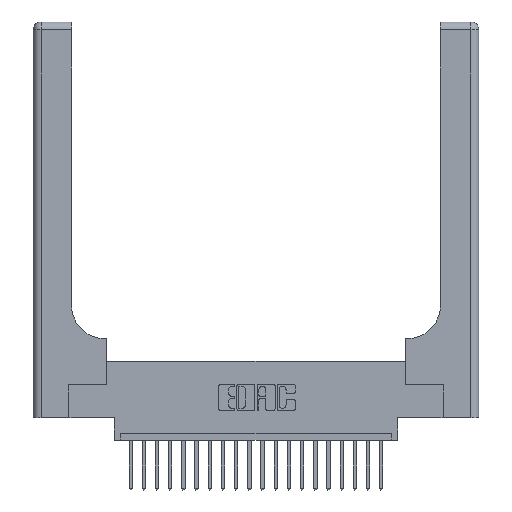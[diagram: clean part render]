
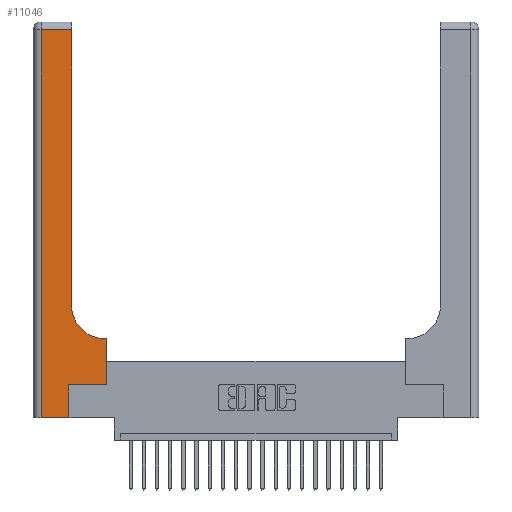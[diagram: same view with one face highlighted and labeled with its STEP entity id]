
A CAD part, top view. The second image highlights one B-rep face of the part: STEP entity #11046.
In plain terms, the highlighted planar face has unit normal (0, 0, 1).
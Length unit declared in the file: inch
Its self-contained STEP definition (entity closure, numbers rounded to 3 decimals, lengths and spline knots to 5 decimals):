
#27 = LINE ( 'NONE', #17472, #4263 ) ;
#276 = EDGE_CURVE ( 'NONE', #8226, #15365, #3996, .T. ) ;
#279 = CARTESIAN_POINT ( 'NONE',  ( 0.269, 0., 0.37 ) ) ;
#427 = CARTESIAN_POINT ( 'NONE',  ( 0.269, 0., 0.37 ) ) ;
#1130 = CARTESIAN_POINT ( 'NONE',  ( 0.2915, 0.6, 0.37 ) ) ;
#1135 = LINE ( 'NONE', #21143, #7682 ) ;
#1364 = EDGE_CURVE ( 'NONE', #17051, #12651, #27, .T. ) ;
#1678 = CARTESIAN_POINT ( 'NONE',  ( 0.5415, 0.85, 0.37 ) ) ;
#1779 = ORIENTED_EDGE ( 'NONE', *, *, #19522, .T. ) ;
#1780 = EDGE_CURVE ( 'NONE', #22300, #11997, #6833, .T. ) ;
#1818 = CARTESIAN_POINT ( 'NONE',  ( 0.5585, 0.25, 0.37 ) ) ;
#1887 = LINE ( 'NONE', #15063, #18547 ) ;
#1990 = FACE_OUTER_BOUND ( 'NONE', #19622, .T. ) ;
#3239 = CARTESIAN_POINT ( 'NONE',  ( 0.06, 2.94, 0.37 ) ) ;
#3416 = DIRECTION ( 'NONE',  ( 0., 1., 0. ) ) ;
#3587 = EDGE_CURVE ( 'NONE', #15365, #22300, #7029, .T. ) ;
#3996 = LINE ( 'NONE', #21252, #12511 ) ;
#4047 = LINE ( 'NONE', #5181, #6327 ) ;
#4263 = VECTOR ( 'NONE', #21125, 39.37008 ) ;
#5181 = CARTESIAN_POINT ( 'NONE',  ( 0.2915, 3., 0.37 ) ) ;
#5636 = CARTESIAN_POINT ( 'NONE',  ( 0.2915, 2.94, 0.37 ) ) ;
#5704 = DIRECTION ( 'NONE',  ( 0., 1., 0. ) ) ;
#6146 = ORIENTED_EDGE ( 'NONE', *, *, #16780, .T. ) ;
#6313 = AXIS2_PLACEMENT_3D ( 'NONE', #6791, #19270, #17471 ) ;
#6327 = VECTOR ( 'NONE', #17854, 39.37008 ) ;
#6339 = DIRECTION ( 'NONE',  ( 0., -1., 0. ) ) ;
#6791 = CARTESIAN_POINT ( 'NONE',  ( 0., 3., 0.37 ) ) ;
#6833 = LINE ( 'NONE', #1130, #15251 ) ;
#6924 = VERTEX_POINT ( 'NONE', #427 ) ;
#7029 = LINE ( 'NONE', #1818, #11277 ) ;
#7682 = VECTOR ( 'NONE', #23117, 39.37008 ) ;
#8226 = VERTEX_POINT ( 'NONE', #12507 ) ;
#8432 = PLANE ( 'NONE',  #6313 ) ;
#8468 = ORIENTED_EDGE ( 'NONE', *, *, #20614, .T. ) ;
#8823 = AXIS2_PLACEMENT_3D ( 'NONE', #1678, #21291, #10594 ) ;
#9630 = DIRECTION ( 'NONE',  ( -1., 0., 0. ) ) ;
#10594 = DIRECTION ( 'NONE',  ( 1., 0., 0. ) ) ;
#11046 = ADVANCED_FACE ( 'NONE', ( #1990 ), #8432, .F. ) ;
#11277 = VECTOR ( 'NONE', #3416, 39.37008 ) ;
#11372 = LINE ( 'NONE', #279, #16965 ) ;
#11997 = VERTEX_POINT ( 'NONE', #13775 ) ;
#12507 = CARTESIAN_POINT ( 'NONE',  ( 0.269, 0.25, 0.37 ) ) ;
#12511 = VECTOR ( 'NONE', #19793, 39.37008 ) ;
#12651 = VERTEX_POINT ( 'NONE', #3239 ) ;
#13613 = EDGE_CURVE ( 'NONE', #19655, #6924, #1135, .T. ) ;
#13775 = CARTESIAN_POINT ( 'NONE',  ( 0.5415, 0.6, 0.37 ) ) ;
#14710 = ORIENTED_EDGE ( 'NONE', *, *, #13613, .T. ) ;
#15063 = CARTESIAN_POINT ( 'NONE',  ( 0.06, 3., 0.37 ) ) ;
#15159 = ORIENTED_EDGE ( 'NONE', *, *, #1780, .T. ) ;
#15251 = VECTOR ( 'NONE', #9630, 39.37008 ) ;
#15365 = VERTEX_POINT ( 'NONE', #21954 ) ;
#15430 = CIRCLE ( 'NONE', #8823, 0.25 ) ;
#15590 = EDGE_CURVE ( 'NONE', #12651, #19655, #1887, .T. ) ;
#16780 = EDGE_CURVE ( 'NONE', #11997, #19632, #15430, .T. ) ;
#16965 = VECTOR ( 'NONE', #5704, 39.37008 ) ;
#17051 = VERTEX_POINT ( 'NONE', #5636 ) ;
#17471 = DIRECTION ( 'NONE',  ( -1., 0., 0. ) ) ;
#17472 = CARTESIAN_POINT ( 'NONE',  ( 0., 2.94, 0.37 ) ) ;
#17854 = DIRECTION ( 'NONE',  ( 0., 1., 0. ) ) ;
#18312 = ORIENTED_EDGE ( 'NONE', *, *, #15590, .T. ) ;
#18547 = VECTOR ( 'NONE', #6339, 39.37008 ) ;
#18673 = ORIENTED_EDGE ( 'NONE', *, *, #276, .T. ) ;
#18733 = CARTESIAN_POINT ( 'NONE',  ( 0.2915, 0.85, 0.37 ) ) ;
#18782 = ORIENTED_EDGE ( 'NONE', *, *, #3587, .T. ) ;
#19270 = DIRECTION ( 'NONE',  ( 0., 0., -1. ) ) ;
#19522 = EDGE_CURVE ( 'NONE', #6924, #8226, #11372, .T. ) ;
#19622 = EDGE_LOOP ( 'NONE', ( #8468, #23241, #18312, #14710, #1779, #18673, #18782, #15159, #6146 ) ) ;
#19632 = VERTEX_POINT ( 'NONE', #18733 ) ;
#19655 = VERTEX_POINT ( 'NONE', #22168 ) ;
#19793 = DIRECTION ( 'NONE',  ( 1., 0., 0. ) ) ;
#20614 = EDGE_CURVE ( 'NONE', #19632, #17051, #4047, .T. ) ;
#21125 = DIRECTION ( 'NONE',  ( -1., 0., 0. ) ) ;
#21143 = CARTESIAN_POINT ( 'NONE',  ( 0., 0., 0.37 ) ) ;
#21236 = CARTESIAN_POINT ( 'NONE',  ( 0.5585, 0.6, 0.37 ) ) ;
#21252 = CARTESIAN_POINT ( 'NONE',  ( 0.269, 0.25, 0.37 ) ) ;
#21291 = DIRECTION ( 'NONE',  ( 0., 0., -1. ) ) ;
#21954 = CARTESIAN_POINT ( 'NONE',  ( 0.5585, 0.25, 0.37 ) ) ;
#22168 = CARTESIAN_POINT ( 'NONE',  ( 0.06, 0., 0.37 ) ) ;
#22300 = VERTEX_POINT ( 'NONE', #21236 ) ;
#23117 = DIRECTION ( 'NONE',  ( 1., 0., 0. ) ) ;
#23241 = ORIENTED_EDGE ( 'NONE', *, *, #1364, .T. ) ;
